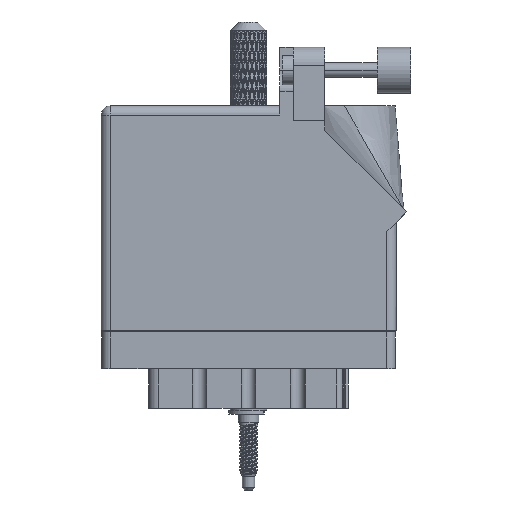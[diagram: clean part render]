
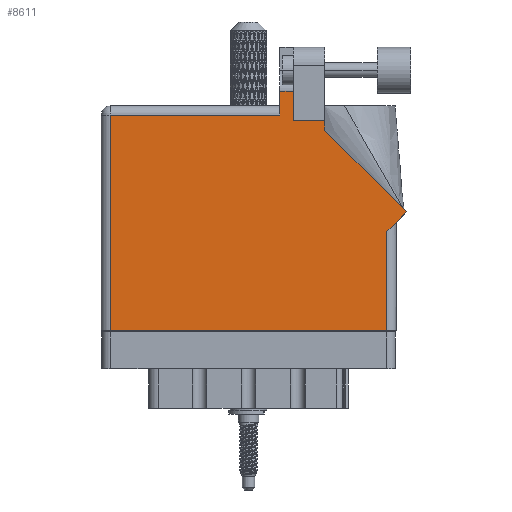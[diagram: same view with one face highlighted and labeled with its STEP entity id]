
A CAD part, front view. The second image highlights one B-rep face of the part: STEP entity #8611.
In plain terms, the highlighted face is planar.
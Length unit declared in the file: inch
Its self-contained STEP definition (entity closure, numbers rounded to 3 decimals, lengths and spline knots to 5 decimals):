
#491 = ORIENTED_EDGE ( 'NONE', *, *, #29363, .T. ) ;
#2190 = CARTESIAN_POINT ( 'NONE',  ( 2.01, 0.737, 0. ) ) ;
#2278 = DIRECTION ( 'NONE',  ( 0., 0., -1. ) ) ;
#3173 = VECTOR ( 'NONE', #29121, 39.37008 ) ;
#3430 = VERTEX_POINT ( 'NONE', #75789 ) ;
#5885 = LINE ( 'NONE', #73199, #55707 ) ;
#8611 = ADVANCED_FACE ( 'NONE', ( #84642 ), #89109, .F. ) ;
#12832 = CARTESIAN_POINT ( 'NONE',  ( 0.062, 1.468, 0. ) ) ;
#13081 = LINE ( 'NONE', #22492, #3173 ) ;
#14767 = DIRECTION ( 'NONE',  ( 0., -1., 0. ) ) ;
#15265 = ORIENTED_EDGE ( 'NONE', *, *, #82394, .T. ) ;
#16924 = DIRECTION ( 'NONE',  ( 1., 0., 0. ) ) ;
#17811 = LINE ( 'NONE', #58741, #40162 ) ;
#19050 = VERTEX_POINT ( 'NONE', #84543 ) ;
#20521 = VERTEX_POINT ( 'NONE', #85301 ) ;
#21470 = VERTEX_POINT ( 'NONE', #64079 ) ;
#22492 = CARTESIAN_POINT ( 'NONE',  ( 1.524, 1.43, 0. ) ) ;
#22732 = DIRECTION ( 'NONE',  ( 0., -1., 0. ) ) ;
#24033 = DIRECTION ( 'NONE',  ( -0.707, 0.707, 0. ) ) ;
#24843 = EDGE_CURVE ( 'NONE', #97728, #19050, #41244, .T. ) ;
#25514 = ORIENTED_EDGE ( 'NONE', *, *, #91936, .T. ) ;
#25852 = EDGE_LOOP ( 'NONE', ( #51326, #48063, #25514, #56263, #92915, #84069, #79368, #15265, #491, #32877, #73211 ) ) ;
#26799 = LINE ( 'NONE', #2190, #68023 ) ;
#26876 = VECTOR ( 'NONE', #77302, 39.37008 ) ;
#28655 = VERTEX_POINT ( 'NONE', #85620 ) ;
#29121 = DIRECTION ( 'NONE',  ( -1., 0., 0. ) ) ;
#29363 = EDGE_CURVE ( 'NONE', #3430, #99813, #85596, .T. ) ;
#32399 = LINE ( 'NONE', #73703, #33565 ) ;
#32877 = ORIENTED_EDGE ( 'NONE', *, *, #99839, .T. ) ;
#33565 = VECTOR ( 'NONE', #16924, 39.37008 ) ;
#34099 = VERTEX_POINT ( 'NONE', #12832 ) ;
#38750 = CARTESIAN_POINT ( 'NONE',  ( 2.08071, 0.80771, 0. ) ) ;
#39446 = LINE ( 'NONE', #53147, #26876 ) ;
#39805 = CARTESIAN_POINT ( 'NONE',  ( 1.217, 1.53, 0. ) ) ;
#40162 = VECTOR ( 'NONE', #90921, 39.37008 ) ;
#40628 = CARTESIAN_POINT ( 'NONE',  ( 0., 1.53, 0. ) ) ;
#41041 = DIRECTION ( 'NONE',  ( 0., 1., 0. ) ) ;
#41244 = LINE ( 'NONE', #48981, #43697 ) ;
#43697 = VECTOR ( 'NONE', #41041, 39.37008 ) ;
#45420 = CARTESIAN_POINT ( 'NONE',  ( 1.524, 1.36442, 0. ) ) ;
#48063 = ORIENTED_EDGE ( 'NONE', *, *, #81525, .T. ) ;
#48981 = CARTESIAN_POINT ( 'NONE',  ( 1.948, 0.737, 0. ) ) ;
#49530 = VECTOR ( 'NONE', #103361, 39.37008 ) ;
#51326 = ORIENTED_EDGE ( 'NONE', *, *, #71405, .T. ) ;
#51969 = LINE ( 'NONE', #70166, #102061 ) ;
#53147 = CARTESIAN_POINT ( 'NONE',  ( 1.311, 1.43, 0. ) ) ;
#54525 = LINE ( 'NONE', #70870, #49530 ) ;
#55707 = VECTOR ( 'NONE', #82261, 39.37008 ) ;
#56263 = ORIENTED_EDGE ( 'NONE', *, *, #76054, .T. ) ;
#58741 = CARTESIAN_POINT ( 'NONE',  ( 0., 1.468, 0. ) ) ;
#60374 = LINE ( 'NONE', #39805, #75305 ) ;
#64079 = CARTESIAN_POINT ( 'NONE',  ( 1.524, 1.43, 0. ) ) ;
#68023 = VECTOR ( 'NONE', #81340, 39.37008 ) ;
#69628 = CARTESIAN_POINT ( 'NONE',  ( 1.217, 1.6315, 0. ) ) ;
#70030 = AXIS2_PLACEMENT_3D ( 'NONE', #40628, #2278, #96793 ) ;
#70166 = CARTESIAN_POINT ( 'NONE',  ( 0.062, 0., 0. ) ) ;
#70410 = VERTEX_POINT ( 'NONE', #74768 ) ;
#70870 = CARTESIAN_POINT ( 'NONE',  ( 1.524, 1.36442, 0. ) ) ;
#71405 = EDGE_CURVE ( 'NONE', #28655, #20521, #39446, .T. ) ;
#73199 = CARTESIAN_POINT ( 'NONE',  ( 1.64177, 1.6315, 0. ) ) ;
#73211 = ORIENTED_EDGE ( 'NONE', *, *, #73857, .T. ) ;
#73703 = CARTESIAN_POINT ( 'NONE',  ( 0., 0., 0. ) ) ;
#73857 = EDGE_CURVE ( 'NONE', #21470, #28655, #13081, .T. ) ;
#74768 = CARTESIAN_POINT ( 'NONE',  ( 0.062, 0., 0. ) ) ;
#75305 = VECTOR ( 'NONE', #22732, 39.37008 ) ;
#75789 = CARTESIAN_POINT ( 'NONE',  ( 2.08071, 0.80771, 0. ) ) ;
#76054 = EDGE_CURVE ( 'NONE', #77666, #34099, #17811, .T. ) ;
#77302 = DIRECTION ( 'NONE',  ( 0., 1., 0. ) ) ;
#77666 = VERTEX_POINT ( 'NONE', #102771 ) ;
#79368 = ORIENTED_EDGE ( 'NONE', *, *, #24843, .T. ) ;
#81081 = EDGE_CURVE ( 'NONE', #34099, #70410, #51969, .T. ) ;
#81340 = DIRECTION ( 'NONE',  ( 0.707, 0.707, 0. ) ) ;
#81525 = EDGE_CURVE ( 'NONE', #20521, #99363, #5885, .T. ) ;
#82261 = DIRECTION ( 'NONE',  ( -1., 0., 0. ) ) ;
#82394 = EDGE_CURVE ( 'NONE', #19050, #3430, #26799, .T. ) ;
#84069 = ORIENTED_EDGE ( 'NONE', *, *, #97431, .T. ) ;
#84543 = CARTESIAN_POINT ( 'NONE',  ( 1.948, 0.675, 0. ) ) ;
#84642 = FACE_OUTER_BOUND ( 'NONE', #25852, .T. ) ;
#85166 = CARTESIAN_POINT ( 'NONE',  ( 1.948, 0., 0. ) ) ;
#85301 = CARTESIAN_POINT ( 'NONE',  ( 1.311, 1.6315, 0. ) ) ;
#85596 = LINE ( 'NONE', #38750, #86774 ) ;
#85620 = CARTESIAN_POINT ( 'NONE',  ( 1.311, 1.43, 0. ) ) ;
#86774 = VECTOR ( 'NONE', #24033, 39.37008 ) ;
#89109 = PLANE ( 'NONE',  #70030 ) ;
#90921 = DIRECTION ( 'NONE',  ( -1., 0., 0. ) ) ;
#91936 = EDGE_CURVE ( 'NONE', #99363, #77666, #60374, .T. ) ;
#92915 = ORIENTED_EDGE ( 'NONE', *, *, #81081, .T. ) ;
#96793 = DIRECTION ( 'NONE',  ( -1., 0., 0. ) ) ;
#97431 = EDGE_CURVE ( 'NONE', #70410, #97728, #32399, .T. ) ;
#97728 = VERTEX_POINT ( 'NONE', #85166 ) ;
#99363 = VERTEX_POINT ( 'NONE', #69628 ) ;
#99813 = VERTEX_POINT ( 'NONE', #45420 ) ;
#99839 = EDGE_CURVE ( 'NONE', #99813, #21470, #54525, .T. ) ;
#102061 = VECTOR ( 'NONE', #14767, 39.37008 ) ;
#102771 = CARTESIAN_POINT ( 'NONE',  ( 1.217, 1.468, 0. ) ) ;
#103361 = DIRECTION ( 'NONE',  ( 0., 1., 0. ) ) ;
